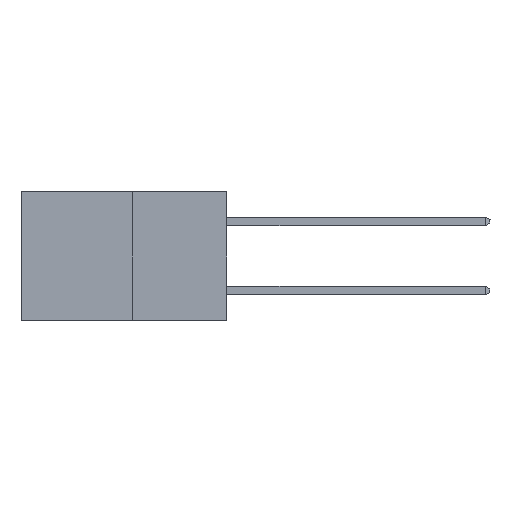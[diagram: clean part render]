
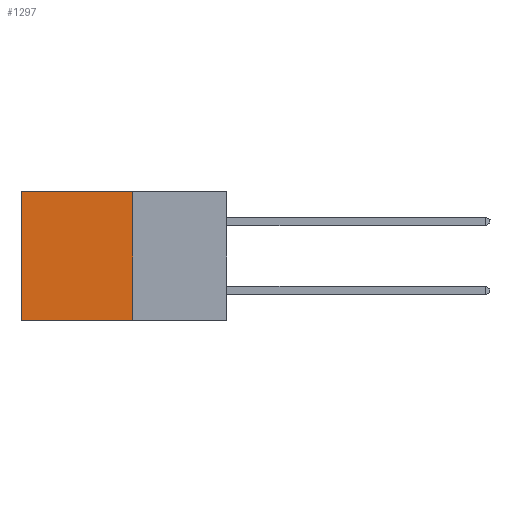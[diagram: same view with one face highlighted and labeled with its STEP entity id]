
A CAD part, left-side view. The second image highlights one B-rep face of the part: STEP entity #1297.
In plain terms, the highlighted planar face has unit normal (-1, 0, 0).
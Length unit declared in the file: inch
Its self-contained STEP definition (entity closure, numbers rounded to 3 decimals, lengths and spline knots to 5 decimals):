
#631 = CARTESIAN_POINT ( 'NONE',  ( 0.277, 0.27, 0. ) ) ;
#1125 = DIRECTION ( 'NONE',  ( 0., 0., -1. ) ) ;
#1297 = ADVANCED_FACE ( 'NONE', ( #26631 ), #17175, .F. ) ;
#2473 = CARTESIAN_POINT ( 'NONE',  ( 0.277, 0.27, -0.37 ) ) ;
#4417 = LINE ( 'NONE', #28617, #31200 ) ;
#4918 = EDGE_CURVE ( 'NONE', #9617, #13821, #12397, .T. ) ;
#5570 = EDGE_CURVE ( 'NONE', #30137, #9617, #4417, .T. ) ;
#5757 = DIRECTION ( 'NONE',  ( 0., 1., 0. ) ) ;
#5976 = CARTESIAN_POINT ( 'NONE',  ( 0.277, 0.27, -0.37 ) ) ;
#8586 = DIRECTION ( 'NONE',  ( 0., 0., -1. ) ) ;
#9247 = EDGE_CURVE ( 'NONE', #23362, #13821, #17676, .T. ) ;
#9617 = VERTEX_POINT ( 'NONE', #17940 ) ;
#10963 = EDGE_LOOP ( 'NONE', ( #18925, #25004, #19232, #26619 ) ) ;
#11148 = CARTESIAN_POINT ( 'NONE',  ( 0.277, 0.59, -0.37 ) ) ;
#11714 = CARTESIAN_POINT ( 'NONE',  ( 0.277, 0.59, -0.37 ) ) ;
#12397 = LINE ( 'NONE', #5976, #17579 ) ;
#13107 = AXIS2_PLACEMENT_3D ( 'NONE', #2473, #22896, #8586 ) ;
#13821 = VERTEX_POINT ( 'NONE', #11714 ) ;
#15214 = CARTESIAN_POINT ( 'NONE',  ( 0.277, 0.27, 0. ) ) ;
#16466 = EDGE_CURVE ( 'NONE', #30137, #23362, #18700, .T. ) ;
#17096 = VECTOR ( 'NONE', #17797, 39.37008 ) ;
#17175 = PLANE ( 'NONE',  #13107 ) ;
#17579 = VECTOR ( 'NONE', #5757, 39.37008 ) ;
#17676 = LINE ( 'NONE', #11148, #23606 ) ;
#17797 = DIRECTION ( 'NONE',  ( 0., 1., 0. ) ) ;
#17940 = CARTESIAN_POINT ( 'NONE',  ( 0.277, 0.27, -0.37 ) ) ;
#18700 = LINE ( 'NONE', #15214, #17096 ) ;
#18925 = ORIENTED_EDGE ( 'NONE', *, *, #9247, .T. ) ;
#19232 = ORIENTED_EDGE ( 'NONE', *, *, #5570, .F. ) ;
#22896 = DIRECTION ( 'NONE',  ( 1., 0., 0. ) ) ;
#23362 = VERTEX_POINT ( 'NONE', #30760 ) ;
#23606 = VECTOR ( 'NONE', #1125, 39.37008 ) ;
#25004 = ORIENTED_EDGE ( 'NONE', *, *, #4918, .F. ) ;
#26619 = ORIENTED_EDGE ( 'NONE', *, *, #16466, .T. ) ;
#26631 = FACE_OUTER_BOUND ( 'NONE', #10963, .T. ) ;
#28522 = DIRECTION ( 'NONE',  ( 0., 0., -1. ) ) ;
#28617 = CARTESIAN_POINT ( 'NONE',  ( 0.277, 0.27, -0.37 ) ) ;
#30137 = VERTEX_POINT ( 'NONE', #631 ) ;
#30760 = CARTESIAN_POINT ( 'NONE',  ( 0.277, 0.59, 0. ) ) ;
#31200 = VECTOR ( 'NONE', #28522, 39.37008 ) ;
